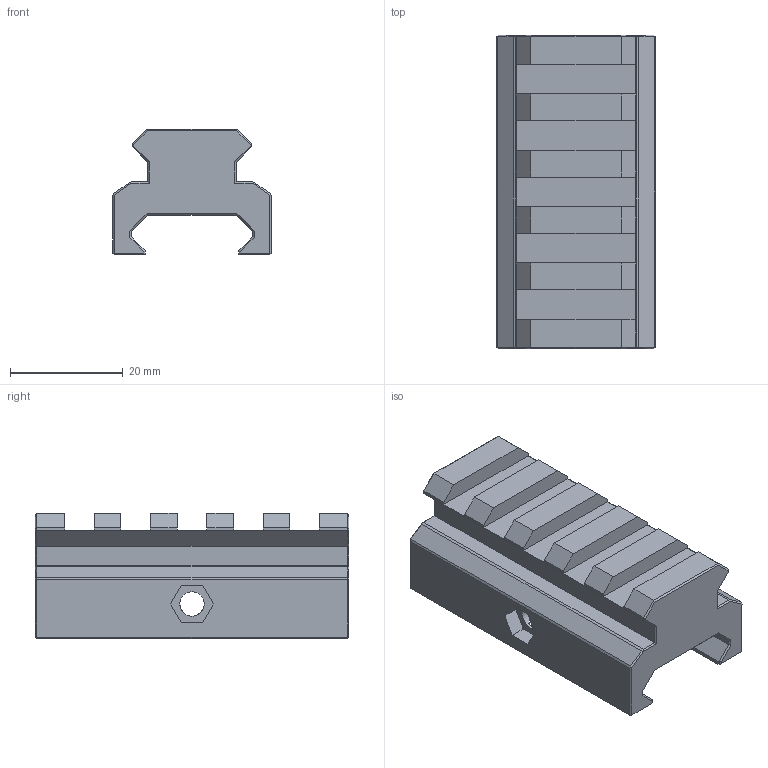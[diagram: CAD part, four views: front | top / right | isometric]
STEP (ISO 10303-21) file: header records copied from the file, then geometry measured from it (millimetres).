
FILE_DESCRIPTION(/* description */ (''),/* implementation_level */ '2;1');
FILE_NAME(/* name */ '15mm Picatinny Riser.step',/* time_stamp */ '2020-03-29T10:47:09-05:00',/* author */ (''),/* organization */ (''),/* preprocessor_version */ 'ST-DEVELOPER v18',/* originating_system */ 'Autodesk Translation Framework v8.12.0.6',/* authorisation */ '');
FILE_SCHEMA (('AUTOMOTIVE_DESIGN { 1 0 10303 214 3 1 1 }'));
Length unit declared in the file: millimetre
Products named in the file (1): Vortex Venom Riser
Bounding box: 28.19 x 55.73 x 22.21 mm (x, y, z)
Volume: 19778.7 mm3; surface area: 8051.6 mm2
Topology: 1 solids, 1 shells, 142 faces, 344 edges, 204 vertices
Faces by surface type: plane 140, cylinder 2
Full cylindrical faces by diameter (mm): 4.318 x1, 7.112 x1
Entity records: 4013 total; most frequent: CARTESIAN_POINT 691, ORIENTED_EDGE 688, DIRECTION 642, EDGE_CURVE 344, LINE 332, VECTOR 332, VERTEX_POINT 204, AXIS2_PLACEMENT_3D 155
